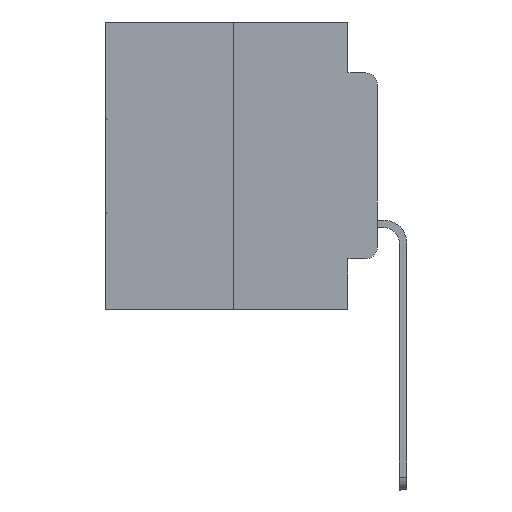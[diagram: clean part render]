
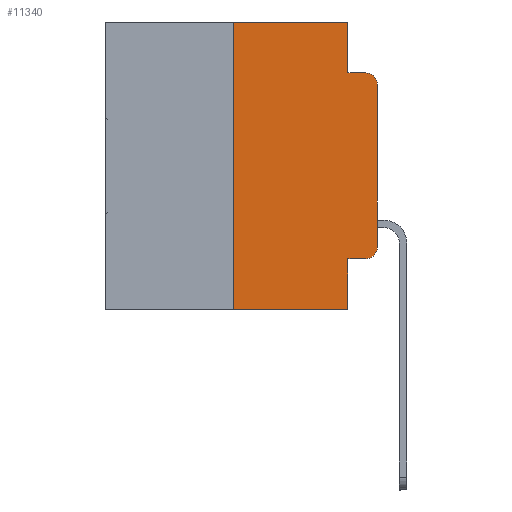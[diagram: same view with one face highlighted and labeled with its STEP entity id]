
A CAD part, left-side view. The second image highlights one B-rep face of the part: STEP entity #11340.
In plain terms, the highlighted planar face has unit normal (-1, 0, 0).
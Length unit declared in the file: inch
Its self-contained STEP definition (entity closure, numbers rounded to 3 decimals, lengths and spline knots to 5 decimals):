
#185 = ORIENTED_EDGE ( 'NONE', *, *, #20499, .F. ) ;
#502 = LINE ( 'NONE', #12769, #891 ) ;
#820 = CARTESIAN_POINT ( 'NONE',  ( 0., 0.02, -0.4115 ) ) ;
#831 = LINE ( 'NONE', #1092, #5376 ) ;
#891 = VECTOR ( 'NONE', #3116, 39.37008 ) ;
#1023 = CARTESIAN_POINT ( 'NONE',  ( 0., 0.051, -0.4115 ) ) ;
#1092 = CARTESIAN_POINT ( 'NONE',  ( 0., 0.473, -0.5 ) ) ;
#2104 = LINE ( 'NONE', #30462, #30132 ) ;
#2466 = DIRECTION ( 'NONE',  ( 0., 0., 1. ) ) ;
#3116 = DIRECTION ( 'NONE',  ( 0., 0., -1. ) ) ;
#3132 = VECTOR ( 'NONE', #20615, 39.37008 ) ;
#3724 = CARTESIAN_POINT ( 'NONE',  ( 0., 0., -0.3915 ) ) ;
#3933 = CARTESIAN_POINT ( 'NONE',  ( 0., 0.02, -0.1085 ) ) ;
#4298 = CARTESIAN_POINT ( 'NONE',  ( 0., 0.051, -0.0885 ) ) ;
#4863 = ORIENTED_EDGE ( 'NONE', *, *, #7003, .F. ) ;
#5216 = VERTEX_POINT ( 'NONE', #3724 ) ;
#5310 = CARTESIAN_POINT ( 'NONE',  ( 0., 0.051, 0. ) ) ;
#5376 = VECTOR ( 'NONE', #17846, 39.37008 ) ;
#6001 = VERTEX_POINT ( 'NONE', #20275 ) ;
#6007 = DIRECTION ( 'NONE',  ( 0., 0., 1. ) ) ;
#6192 = VECTOR ( 'NONE', #20066, 39.37008 ) ;
#6398 = ORIENTED_EDGE ( 'NONE', *, *, #29407, .T. ) ;
#6556 = ORIENTED_EDGE ( 'NONE', *, *, #29771, .F. ) ;
#7003 = EDGE_CURVE ( 'NONE', #17521, #30539, #22758, .T. ) ;
#7616 = CARTESIAN_POINT ( 'NONE',  ( 0., 0.25, 0. ) ) ;
#7861 = CARTESIAN_POINT ( 'NONE',  ( 0., 0.473, 0. ) ) ;
#8063 = CARTESIAN_POINT ( 'NONE',  ( 0., 0.473, 0. ) ) ;
#8656 = DIRECTION ( 'NONE',  ( -1., 0., 0. ) ) ;
#8964 = ORIENTED_EDGE ( 'NONE', *, *, #30581, .T. ) ;
#9054 = DIRECTION ( 'NONE',  ( 0., 0., -1. ) ) ;
#9873 = VECTOR ( 'NONE', #2466, 39.37008 ) ;
#10433 = EDGE_CURVE ( 'NONE', #10631, #6001, #28140, .T. ) ;
#10631 = VERTEX_POINT ( 'NONE', #30982 ) ;
#10645 = LINE ( 'NONE', #7616, #9873 ) ;
#10974 = DIRECTION ( 'NONE',  ( -1., 0., 0. ) ) ;
#11340 = ADVANCED_FACE ( 'NONE', ( #29906 ), #27073, .F. ) ;
#11398 = DIRECTION ( 'NONE',  ( 0., 0., -1. ) ) ;
#11479 = LINE ( 'NONE', #24998, #17034 ) ;
#11519 = DIRECTION ( 'NONE',  ( 0., 0., -1. ) ) ;
#11897 = AXIS2_PLACEMENT_3D ( 'NONE', #8063, #15134, #29345 ) ;
#12139 = LINE ( 'NONE', #4298, #3132 ) ;
#12243 = EDGE_LOOP ( 'NONE', ( #6398, #30434, #185, #21508, #4863, #16172, #8964, #6556, #22413, #17865 ) ) ;
#12561 = VERTEX_POINT ( 'NONE', #22977 ) ;
#12769 = CARTESIAN_POINT ( 'NONE',  ( 0., 0.051, 0. ) ) ;
#14094 = VERTEX_POINT ( 'NONE', #30892 ) ;
#14280 = AXIS2_PLACEMENT_3D ( 'NONE', #3933, #10974, #11398 ) ;
#14689 = EDGE_CURVE ( 'NONE', #29386, #5216, #20947, .T. ) ;
#15134 = DIRECTION ( 'NONE',  ( 1., 0., 0. ) ) ;
#16172 = ORIENTED_EDGE ( 'NONE', *, *, #30332, .F. ) ;
#17034 = VECTOR ( 'NONE', #6007, 39.37008 ) ;
#17521 = VERTEX_POINT ( 'NONE', #30552 ) ;
#17769 = DIRECTION ( 'NONE',  ( 0., -1., 0. ) ) ;
#17846 = DIRECTION ( 'NONE',  ( 0., -1., 0. ) ) ;
#17865 = ORIENTED_EDGE ( 'NONE', *, *, #14689, .T. ) ;
#17890 = VERTEX_POINT ( 'NONE', #22949 ) ;
#17918 = CARTESIAN_POINT ( 'NONE',  ( 0., 0.051, -0.4115 ) ) ;
#19610 = EDGE_CURVE ( 'NONE', #30539, #12561, #2104, .T. ) ;
#20066 = DIRECTION ( 'NONE',  ( 0., -1., 0. ) ) ;
#20134 = VECTOR ( 'NONE', #17769, 39.37008 ) ;
#20275 = CARTESIAN_POINT ( 'NONE',  ( 0., 0.02, -0.0885 ) ) ;
#20499 = EDGE_CURVE ( 'NONE', #12561, #6001, #12139, .T. ) ;
#20615 = DIRECTION ( 'NONE',  ( 0., -1., 0. ) ) ;
#20620 = EDGE_CURVE ( 'NONE', #26391, #29386, #21531, .T. ) ;
#20947 = CIRCLE ( 'NONE', #27813, 0.02 ) ;
#21508 = ORIENTED_EDGE ( 'NONE', *, *, #19610, .F. ) ;
#21531 = LINE ( 'NONE', #1023, #6192 ) ;
#22413 = ORIENTED_EDGE ( 'NONE', *, *, #20620, .T. ) ;
#22758 = LINE ( 'NONE', #7861, #20134 ) ;
#22949 = CARTESIAN_POINT ( 'NONE',  ( 0., 0.25, -0.5 ) ) ;
#22977 = CARTESIAN_POINT ( 'NONE',  ( 0., 0.051, -0.0885 ) ) ;
#23265 = CARTESIAN_POINT ( 'NONE',  ( 0., 0.02, -0.3915 ) ) ;
#24998 = CARTESIAN_POINT ( 'NONE',  ( 0., 0., 0. ) ) ;
#26391 = VERTEX_POINT ( 'NONE', #17918 ) ;
#27073 = PLANE ( 'NONE',  #11897 ) ;
#27813 = AXIS2_PLACEMENT_3D ( 'NONE', #23265, #8656, #9054 ) ;
#28140 = CIRCLE ( 'NONE', #14280, 0.02 ) ;
#29345 = DIRECTION ( 'NONE',  ( 0., 0., -1. ) ) ;
#29386 = VERTEX_POINT ( 'NONE', #820 ) ;
#29407 = EDGE_CURVE ( 'NONE', #5216, #10631, #11479, .T. ) ;
#29771 = EDGE_CURVE ( 'NONE', #26391, #14094, #502, .T. ) ;
#29906 = FACE_OUTER_BOUND ( 'NONE', #12243, .T. ) ;
#30132 = VECTOR ( 'NONE', #11519, 39.37008 ) ;
#30332 = EDGE_CURVE ( 'NONE', #17890, #17521, #10645, .T. ) ;
#30434 = ORIENTED_EDGE ( 'NONE', *, *, #10433, .T. ) ;
#30462 = CARTESIAN_POINT ( 'NONE',  ( 0., 0.051, 0. ) ) ;
#30539 = VERTEX_POINT ( 'NONE', #5310 ) ;
#30552 = CARTESIAN_POINT ( 'NONE',  ( 0., 0.25, 0. ) ) ;
#30581 = EDGE_CURVE ( 'NONE', #17890, #14094, #831, .T. ) ;
#30892 = CARTESIAN_POINT ( 'NONE',  ( 0., 0.051, -0.5 ) ) ;
#30982 = CARTESIAN_POINT ( 'NONE',  ( 0., 0., -0.1085 ) ) ;
